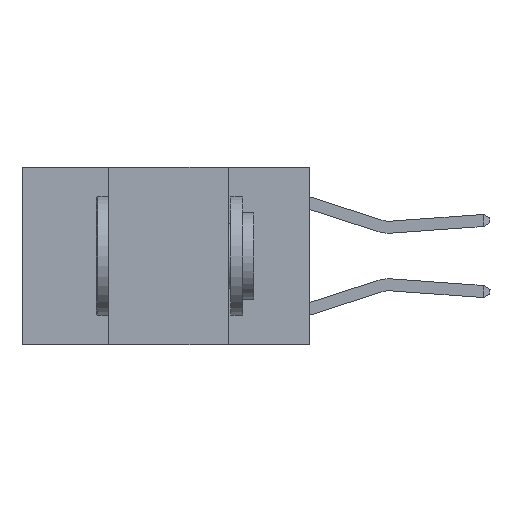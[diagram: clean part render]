
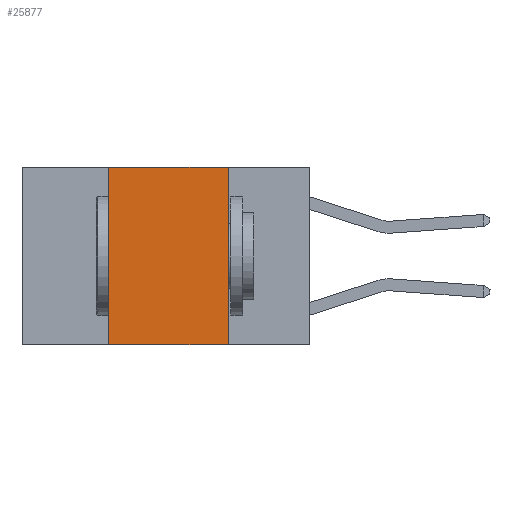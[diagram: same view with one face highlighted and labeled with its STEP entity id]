
A CAD part, left-side view. The second image highlights one B-rep face of the part: STEP entity #25877.
In plain terms, the highlighted planar face has unit normal (-1, 0, 0).
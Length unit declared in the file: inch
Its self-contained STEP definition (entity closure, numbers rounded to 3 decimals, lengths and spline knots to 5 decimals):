
#108 = DIRECTION ( 'NONE',  ( 0., -1., 0. ) ) ;
#278 = EDGE_CURVE ( 'NONE', #822, #6897, #8260, .T. ) ;
#385 = CARTESIAN_POINT ( 'NONE',  ( 0., 0.6, -0.37 ) ) ;
#822 = VERTEX_POINT ( 'NONE', #4554 ) ;
#844 = LINE ( 'NONE', #11666, #3587 ) ;
#1020 = VECTOR ( 'NONE', #2297, 39.37008 ) ;
#2297 = DIRECTION ( 'NONE',  ( 0., 0., -1. ) ) ;
#3561 = DIRECTION ( 'NONE',  ( 1., 0., 0. ) ) ;
#3587 = VECTOR ( 'NONE', #22163, 39.37008 ) ;
#4259 = VERTEX_POINT ( 'NONE', #20647 ) ;
#4554 = CARTESIAN_POINT ( 'NONE',  ( 0., 0.42, -0.37 ) ) ;
#4710 = AXIS2_PLACEMENT_3D ( 'NONE', #26693, #3561, #20405 ) ;
#5031 = VECTOR ( 'NONE', #20736, 39.37008 ) ;
#5292 = ORIENTED_EDGE ( 'NONE', *, *, #11208, .F. ) ;
#6662 = LINE ( 'NONE', #15212, #1020 ) ;
#6897 = VERTEX_POINT ( 'NONE', #19124 ) ;
#8260 = LINE ( 'NONE', #12731, #5031 ) ;
#9739 = PLANE ( 'NONE',  #4710 ) ;
#11208 = EDGE_CURVE ( 'NONE', #6897, #15391, #844, .T. ) ;
#11666 = CARTESIAN_POINT ( 'NONE',  ( 0., 0.6, 0. ) ) ;
#11973 = ORIENTED_EDGE ( 'NONE', *, *, #23043, .F. ) ;
#12731 = CARTESIAN_POINT ( 'NONE',  ( 0., 0.42, 0. ) ) ;
#14175 = ORIENTED_EDGE ( 'NONE', *, *, #278, .F. ) ;
#14226 = FACE_OUTER_BOUND ( 'NONE', #19145, .T. ) ;
#15212 = CARTESIAN_POINT ( 'NONE',  ( 0., 0.17, 0. ) ) ;
#15391 = VERTEX_POINT ( 'NONE', #23805 ) ;
#15397 = EDGE_CURVE ( 'NONE', #822, #4259, #25621, .T. ) ;
#19124 = CARTESIAN_POINT ( 'NONE',  ( 0., 0.42, 0. ) ) ;
#19145 = EDGE_LOOP ( 'NONE', ( #11973, #5292, #14175, #24122 ) ) ;
#20405 = DIRECTION ( 'NONE',  ( 0., 0., -1. ) ) ;
#20647 = CARTESIAN_POINT ( 'NONE',  ( 0., 0.17, -0.37 ) ) ;
#20736 = DIRECTION ( 'NONE',  ( 0., 0., 1. ) ) ;
#22163 = DIRECTION ( 'NONE',  ( 0., -1., 0. ) ) ;
#22959 = VECTOR ( 'NONE', #108, 39.37008 ) ;
#23043 = EDGE_CURVE ( 'NONE', #15391, #4259, #6662, .T. ) ;
#23805 = CARTESIAN_POINT ( 'NONE',  ( 0., 0.17, 0. ) ) ;
#24122 = ORIENTED_EDGE ( 'NONE', *, *, #15397, .T. ) ;
#25621 = LINE ( 'NONE', #385, #22959 ) ;
#25877 = ADVANCED_FACE ( 'NONE', ( #14226 ), #9739, .F. ) ;
#26693 = CARTESIAN_POINT ( 'NONE',  ( 0., 0.6, 0. ) ) ;
